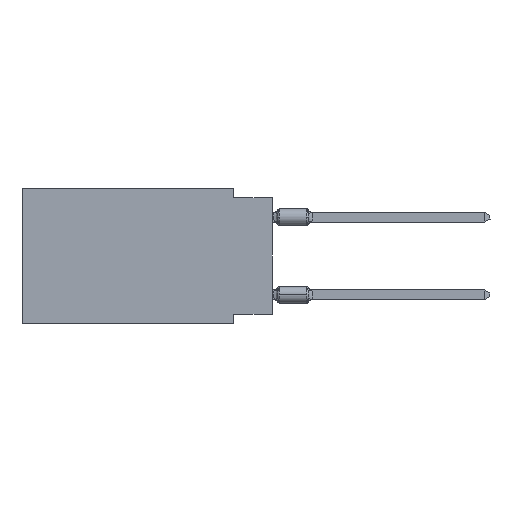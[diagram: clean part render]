
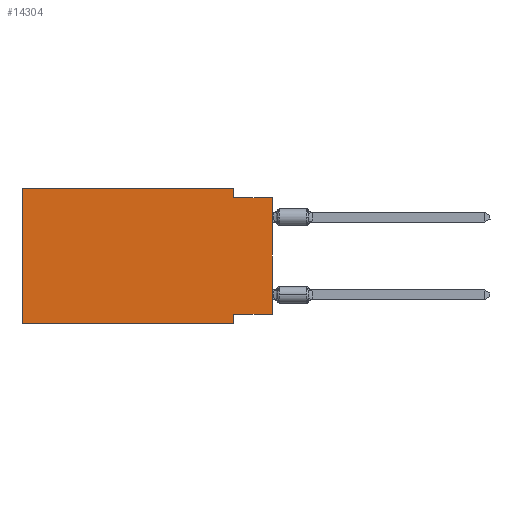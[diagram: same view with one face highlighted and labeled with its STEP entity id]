
A CAD part, left-side view. The second image highlights one B-rep face of the part: STEP entity #14304.
In plain terms, the highlighted planar face has unit normal (-1, 0, 0).
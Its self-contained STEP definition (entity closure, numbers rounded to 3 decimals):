
#503 = CARTESIAN_POINT ( 'NONE',  ( 0., 0., -8.255 ) ) ;
#1866 = EDGE_CURVE ( 'NONE', #37100, #24549, #33826, .T. ) ;
#2442 = EDGE_CURVE ( 'NONE', #15327, #30950, #30301, .T. ) ;
#2843 = CARTESIAN_POINT ( 'NONE',  ( 0., 16.383, 0. ) ) ;
#2903 = DIRECTION ( 'NONE',  ( 0., 1., 0. ) ) ;
#3050 = EDGE_CURVE ( 'NONE', #37100, #15327, #18983, .T. ) ;
#3261 = DIRECTION ( 'NONE',  ( 0., -1., 0. ) ) ;
#3986 = VECTOR ( 'NONE', #2903, 1000. ) ;
#4113 = LINE ( 'NONE', #30570, #9120 ) ;
#5015 = DIRECTION ( 'NONE',  ( 1., 0., 0. ) ) ;
#6637 = ORIENTED_EDGE ( 'NONE', *, *, #40079, .F. ) ;
#8261 = PLANE ( 'NONE',  #20720 ) ;
#8887 = VERTEX_POINT ( 'NONE', #11601 ) ;
#9071 = LINE ( 'NONE', #18625, #22509 ) ;
#9120 = VECTOR ( 'NONE', #34021, 1000. ) ;
#9464 = VECTOR ( 'NONE', #10584, 1000. ) ;
#10194 = LINE ( 'NONE', #2843, #38400 ) ;
#10584 = DIRECTION ( 'NONE',  ( 0., 0., -1. ) ) ;
#11245 = VERTEX_POINT ( 'NONE', #19244 ) ;
#11601 = CARTESIAN_POINT ( 'NONE',  ( 0., 2.54, -0.635 ) ) ;
#11701 = VERTEX_POINT ( 'NONE', #29101 ) ;
#12740 = CARTESIAN_POINT ( 'NONE',  ( 0., 2.54, -8.89 ) ) ;
#13200 = LINE ( 'NONE', #26425, #38212 ) ;
#13845 = CARTESIAN_POINT ( 'NONE',  ( 0., 2.54, -8.89 ) ) ;
#14304 = ADVANCED_FACE ( 'NONE', ( #34485 ), #8261, .F. ) ;
#15327 = VERTEX_POINT ( 'NONE', #17038 ) ;
#17038 = CARTESIAN_POINT ( 'NONE',  ( 0., 2.54, -8.255 ) ) ;
#18259 = DIRECTION ( 'NONE',  ( 0., 0., -1. ) ) ;
#18625 = CARTESIAN_POINT ( 'NONE',  ( 0., 16.383, 0. ) ) ;
#18983 = LINE ( 'NONE', #32600, #3986 ) ;
#19244 = CARTESIAN_POINT ( 'NONE',  ( 0., 16.383, 0. ) ) ;
#20650 = LINE ( 'NONE', #33847, #20825 ) ;
#20720 = AXIS2_PLACEMENT_3D ( 'NONE', #34702, #5015, #18259 ) ;
#20825 = VECTOR ( 'NONE', #30610, 1000. ) ;
#21856 = ORIENTED_EDGE ( 'NONE', *, *, #29579, .F. ) ;
#22509 = VECTOR ( 'NONE', #32042, 1000. ) ;
#23034 = CARTESIAN_POINT ( 'NONE',  ( 0., 2.54, 0. ) ) ;
#23289 = ORIENTED_EDGE ( 'NONE', *, *, #38589, .F. ) ;
#24053 = ORIENTED_EDGE ( 'NONE', *, *, #2442, .F. ) ;
#24065 = ORIENTED_EDGE ( 'NONE', *, *, #1866, .T. ) ;
#24549 = VERTEX_POINT ( 'NONE', #39305 ) ;
#26425 = CARTESIAN_POINT ( 'NONE',  ( 0., 16.383, -8.89 ) ) ;
#26908 = DIRECTION ( 'NONE',  ( 0., 0., 1. ) ) ;
#27108 = VERTEX_POINT ( 'NONE', #23034 ) ;
#28138 = VECTOR ( 'NONE', #26908, 1000. ) ;
#28198 = EDGE_CURVE ( 'NONE', #11245, #27108, #10194, .T. ) ;
#29101 = CARTESIAN_POINT ( 'NONE',  ( 0., 16.383, -8.89 ) ) ;
#29421 = ORIENTED_EDGE ( 'NONE', *, *, #40450, .T. ) ;
#29579 = EDGE_CURVE ( 'NONE', #11701, #11245, #9071, .T. ) ;
#30301 = LINE ( 'NONE', #13845, #9464 ) ;
#30325 = EDGE_LOOP ( 'NONE', ( #24065, #6637, #23289, #39396, #21856, #29421, #24053, #34159 ) ) ;
#30570 = CARTESIAN_POINT ( 'NONE',  ( 0., 0., -0.635 ) ) ;
#30610 = DIRECTION ( 'NONE',  ( 0., 0., -1. ) ) ;
#30950 = VERTEX_POINT ( 'NONE', #12740 ) ;
#32042 = DIRECTION ( 'NONE',  ( 0., 0., 1. ) ) ;
#32600 = CARTESIAN_POINT ( 'NONE',  ( 0., 0., -8.255 ) ) ;
#33826 = LINE ( 'NONE', #34042, #28138 ) ;
#33847 = CARTESIAN_POINT ( 'NONE',  ( 0., 2.54, 0. ) ) ;
#34021 = DIRECTION ( 'NONE',  ( 0., -1., 0. ) ) ;
#34042 = CARTESIAN_POINT ( 'NONE',  ( 0., 0., 0. ) ) ;
#34159 = ORIENTED_EDGE ( 'NONE', *, *, #3050, .F. ) ;
#34485 = FACE_OUTER_BOUND ( 'NONE', #30325, .T. ) ;
#34702 = CARTESIAN_POINT ( 'NONE',  ( 0., 16.383, 0. ) ) ;
#37100 = VERTEX_POINT ( 'NONE', #503 ) ;
#38212 = VECTOR ( 'NONE', #39643, 1000. ) ;
#38400 = VECTOR ( 'NONE', #3261, 1000. ) ;
#38589 = EDGE_CURVE ( 'NONE', #27108, #8887, #20650, .T. ) ;
#39305 = CARTESIAN_POINT ( 'NONE',  ( 0., 0., -0.635 ) ) ;
#39396 = ORIENTED_EDGE ( 'NONE', *, *, #28198, .F. ) ;
#39643 = DIRECTION ( 'NONE',  ( 0., -1., 0. ) ) ;
#40079 = EDGE_CURVE ( 'NONE', #8887, #24549, #4113, .T. ) ;
#40450 = EDGE_CURVE ( 'NONE', #11701, #30950, #13200, .T. ) ;
